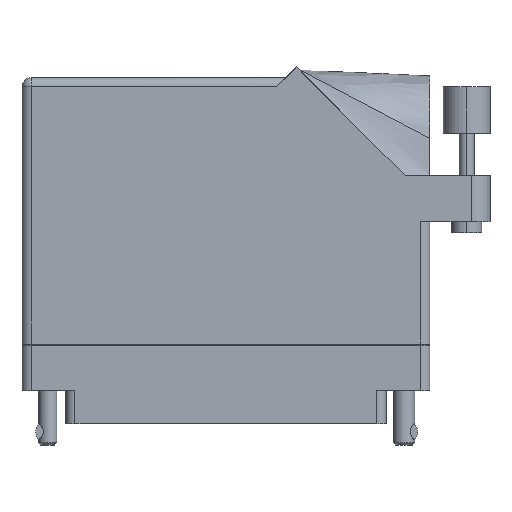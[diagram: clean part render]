
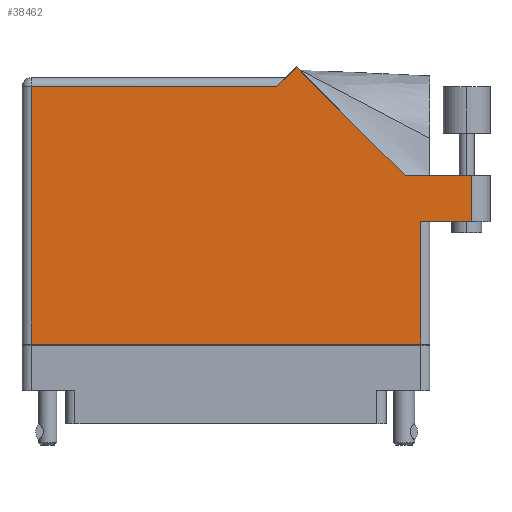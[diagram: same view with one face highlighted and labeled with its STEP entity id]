
A CAD part, front view. The second image highlights one B-rep face of the part: STEP entity #38462.
In plain terms, the highlighted face is planar.
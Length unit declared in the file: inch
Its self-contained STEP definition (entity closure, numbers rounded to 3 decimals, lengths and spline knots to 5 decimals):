
#262 = DIRECTION ( 'NONE',  ( 0., 1., 0. ) ) ;
#278 = DIRECTION ( 'NONE',  ( -1., 0., 0. ) ) ;
#5176 = CARTESIAN_POINT ( 'NONE',  ( 1.359, 0.715, 0.617 ) ) ;
#7176 = ORIENTED_EDGE ( 'NONE', *, *, #67998, .T. ) ;
#10255 = EDGE_CURVE ( 'NONE', #50780, #31364, #77185, .T. ) ;
#12776 = DIRECTION ( 'NONE',  ( -1., 0., 0. ) ) ;
#13494 = PLANE ( 'NONE',  #52727 ) ;
#13532 = ORIENTED_EDGE ( 'NONE', *, *, #24649, .T. ) ;
#13883 = DIRECTION ( 'NONE',  ( 1., 0., 0. ) ) ;
#14179 = CARTESIAN_POINT ( 'NONE',  ( 0.337, 1.613, 0.617 ) ) ;
#14281 = DIRECTION ( 'NONE',  ( -1., 0., 0. ) ) ;
#16579 = VERTEX_POINT ( 'NONE', #42399 ) ;
#16786 = VECTOR ( 'NONE', #12776, 39.37008 ) ;
#19902 = ORIENTED_EDGE ( 'NONE', *, *, #54154, .T. ) ;
#20234 = CARTESIAN_POINT ( 'NONE',  ( 1.297, -0.1, 0.617 ) ) ;
#20397 = VECTOR ( 'NONE', #58148, 39.37008 ) ;
#20430 = CARTESIAN_POINT ( 'NONE',  ( 0.399, 1.675, 0.617 ) ) ;
#20725 = LINE ( 'NONE', #67943, #59519 ) ;
#20796 = LINE ( 'NONE', #54669, #42588 ) ;
#22783 = VERTEX_POINT ( 'NONE', #31143 ) ;
#24649 = EDGE_CURVE ( 'NONE', #22783, #39217, #36987, .T. ) ;
#24863 = DIRECTION ( 'NONE',  ( 0., 1., 0. ) ) ;
#26465 = EDGE_CURVE ( 'NONE', #58899, #55704, #29013, .T. ) ;
#27102 = CARTESIAN_POINT ( 'NONE',  ( 1.634, 1.022, 0.617 ) ) ;
#29013 = LINE ( 'NONE', #30690, #16786 ) ;
#30651 = ORIENTED_EDGE ( 'NONE', *, *, #54930, .T. ) ;
#30690 = CARTESIAN_POINT ( 'NONE',  ( 1.759, 1.022, 0.617 ) ) ;
#31143 = CARTESIAN_POINT ( 'NONE',  ( -1.297, -0.1, 0.617 ) ) ;
#31363 = CARTESIAN_POINT ( 'NONE',  ( 1.297, 0.715, 0.617 ) ) ;
#31364 = VERTEX_POINT ( 'NONE', #33462 ) ;
#32748 = DIRECTION ( 'NONE',  ( 0., -1., 0. ) ) ;
#33462 = CARTESIAN_POINT ( 'NONE',  ( 1.634, 0.715, 0.617 ) ) ;
#35516 = DIRECTION ( 'NONE',  ( 1., 0., 0. ) ) ;
#36987 = LINE ( 'NONE', #69403, #58711 ) ;
#38462 = ADVANCED_FACE ( 'NONE', ( #54289 ), #13494, .F. ) ;
#39217 = VERTEX_POINT ( 'NONE', #20234 ) ;
#40292 = LINE ( 'NONE', #31363, #56295 ) ;
#41123 = LINE ( 'NONE', #20430, #54278 ) ;
#42399 = CARTESIAN_POINT ( 'NONE',  ( 0.46971, 1.74571, 0.617 ) ) ;
#42588 = VECTOR ( 'NONE', #278, 39.37008 ) ;
#44761 = CARTESIAN_POINT ( 'NONE',  ( 1.19342, 1.022, 0.617 ) ) ;
#47283 = VERTEX_POINT ( 'NONE', #14179 ) ;
#47849 = ORIENTED_EDGE ( 'NONE', *, *, #50273, .T. ) ;
#49492 = CARTESIAN_POINT ( 'NONE',  ( 1.634, 1.022, 0.617 ) ) ;
#50273 = EDGE_CURVE ( 'NONE', #16579, #47283, #41123, .T. ) ;
#50780 = VERTEX_POINT ( 'NONE', #63073 ) ;
#52427 = ORIENTED_EDGE ( 'NONE', *, *, #10255, .T. ) ;
#52727 = AXIS2_PLACEMENT_3D ( 'NONE', #68770, #68506, #14281 ) ;
#52902 = EDGE_LOOP ( 'NONE', ( #52427, #19902, #71344, #65376, #47849, #7176, #55386, #13532, #30651 ) ) ;
#53946 = EDGE_CURVE ( 'NONE', #55704, #16579, #64877, .T. ) ;
#54154 = EDGE_CURVE ( 'NONE', #31364, #58899, #61113, .T. ) ;
#54278 = VECTOR ( 'NONE', #75772, 39.37008 ) ;
#54289 = FACE_OUTER_BOUND ( 'NONE', #52902, .T. ) ;
#54669 = CARTESIAN_POINT ( 'NONE',  ( -1.359, 1.613, 0.617 ) ) ;
#54930 = EDGE_CURVE ( 'NONE', #39217, #50780, #40292, .T. ) ;
#55386 = ORIENTED_EDGE ( 'NONE', *, *, #61127, .T. ) ;
#55704 = VERTEX_POINT ( 'NONE', #44761 ) ;
#56295 = VECTOR ( 'NONE', #262, 39.37008 ) ;
#56459 = CARTESIAN_POINT ( 'NONE',  ( -1.297, 1.613, 0.617 ) ) ;
#58148 = DIRECTION ( 'NONE',  ( -0.707, 0.707, 0. ) ) ;
#58711 = VECTOR ( 'NONE', #13883, 39.37008 ) ;
#58899 = VERTEX_POINT ( 'NONE', #27102 ) ;
#59113 = VECTOR ( 'NONE', #35516, 39.37008 ) ;
#59519 = VECTOR ( 'NONE', #32748, 39.37008 ) ;
#61113 = LINE ( 'NONE', #49492, #73501 ) ;
#61127 = EDGE_CURVE ( 'NONE', #75617, #22783, #20725, .T. ) ;
#63073 = CARTESIAN_POINT ( 'NONE',  ( 1.297, 0.715, 0.617 ) ) ;
#64877 = LINE ( 'NONE', #76724, #20397 ) ;
#65376 = ORIENTED_EDGE ( 'NONE', *, *, #53946, .T. ) ;
#67943 = CARTESIAN_POINT ( 'NONE',  ( -1.297, -0.1, 0.617 ) ) ;
#67998 = EDGE_CURVE ( 'NONE', #47283, #75617, #20796, .T. ) ;
#68506 = DIRECTION ( 'NONE',  ( 0., 0., -1. ) ) ;
#68770 = CARTESIAN_POINT ( 'NONE',  ( -1.359, 1.675, 0.617 ) ) ;
#69403 = CARTESIAN_POINT ( 'NONE',  ( -1.359, -0.1, 0.617 ) ) ;
#71344 = ORIENTED_EDGE ( 'NONE', *, *, #26465, .T. ) ;
#73501 = VECTOR ( 'NONE', #24863, 39.37008 ) ;
#75617 = VERTEX_POINT ( 'NONE', #56459 ) ;
#75772 = DIRECTION ( 'NONE',  ( -0.707, -0.707, 0. ) ) ;
#76724 = CARTESIAN_POINT ( 'NONE',  ( 1.19342, 1.022, 0.617 ) ) ;
#77185 = LINE ( 'NONE', #5176, #59113 ) ;
